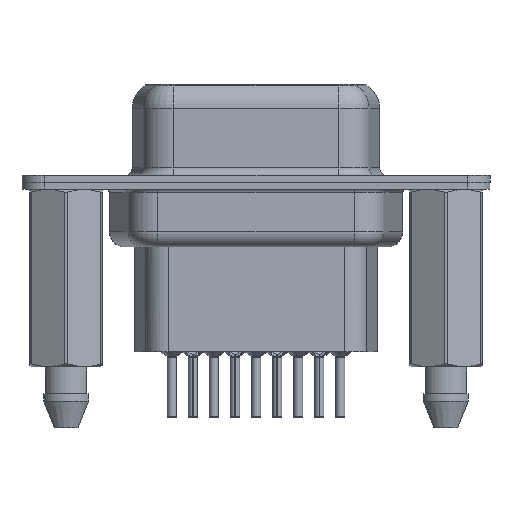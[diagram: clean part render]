
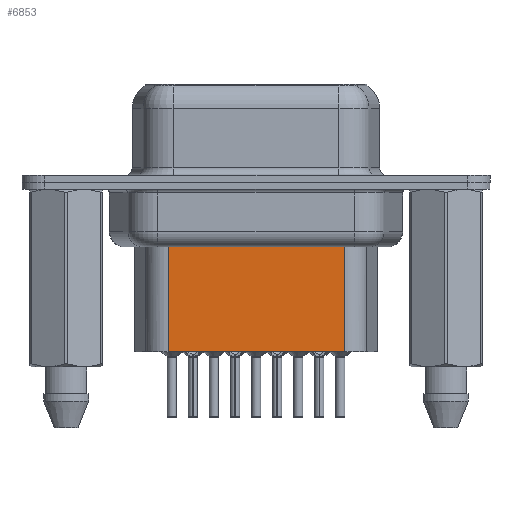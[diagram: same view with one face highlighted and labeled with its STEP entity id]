
A CAD part, front view. The second image highlights one B-rep face of the part: STEP entity #6853.
In plain terms, the highlighted planar face has unit normal (0, -1, 0).
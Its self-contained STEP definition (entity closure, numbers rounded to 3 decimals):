
#758 = CARTESIAN_POINT ( 'NONE',  ( 6.706, -3.5, -4.097 ) ) ;
#928 = CARTESIAN_POINT ( 'NONE',  ( 6.706, -3.5, -3.1 ) ) ;
#2281 = EDGE_CURVE ( 'NONE', #19360, #7440, #21546, .T. ) ;
#2859 = AXIS2_PLACEMENT_3D ( 'NONE', #928, #18677, #21998 ) ;
#3710 = ORIENTED_EDGE ( 'NONE', *, *, #4539, .T. ) ;
#3723 = DIRECTION ( 'NONE',  ( -1., 0., 0. ) ) ;
#4539 = EDGE_CURVE ( 'NONE', #7440, #18703, #18444, .T. ) ;
#6853 = ADVANCED_FACE ( 'NONE', ( #16727 ), #15343, .T. ) ;
#7440 = VERTEX_POINT ( 'NONE', #758 ) ;
#7667 = LINE ( 'NONE', #19545, #13420 ) ;
#11241 = CARTESIAN_POINT ( 'NONE',  ( 6.706, -3.5, -11.15 ) ) ;
#12076 = VECTOR ( 'NONE', #21766, 1000. ) ;
#12569 = VERTEX_POINT ( 'NONE', #12985 ) ;
#12985 = CARTESIAN_POINT ( 'NONE',  ( 18.294, -3.5, -11.15 ) ) ;
#13420 = VECTOR ( 'NONE', #3723, 1000. ) ;
#14421 = DIRECTION ( 'NONE',  ( -1., 0., 0. ) ) ;
#14539 = CARTESIAN_POINT ( 'NONE',  ( 6.459, -3.5, -4.097 ) ) ;
#15077 = VECTOR ( 'NONE', #14421, 1000. ) ;
#15098 = ORIENTED_EDGE ( 'NONE', *, *, #2281, .T. ) ;
#15343 = PLANE ( 'NONE',  #2859 ) ;
#16295 = VECTOR ( 'NONE', #19643, 1000. ) ;
#16582 = EDGE_CURVE ( 'NONE', #19360, #12569, #19754, .T. ) ;
#16727 = FACE_OUTER_BOUND ( 'NONE', #22612, .T. ) ;
#17377 = ORIENTED_EDGE ( 'NONE', *, *, #16582, .F. ) ;
#18444 = LINE ( 'NONE', #18986, #12076 ) ;
#18601 = EDGE_CURVE ( 'NONE', #12569, #18703, #7667, .T. ) ;
#18677 = DIRECTION ( 'NONE',  ( 0., -1., 0. ) ) ;
#18703 = VERTEX_POINT ( 'NONE', #11241 ) ;
#18986 = CARTESIAN_POINT ( 'NONE',  ( 6.706, -3.5, -3.1 ) ) ;
#19360 = VERTEX_POINT ( 'NONE', #22179 ) ;
#19545 = CARTESIAN_POINT ( 'NONE',  ( 6.706, -3.5, -11.15 ) ) ;
#19643 = DIRECTION ( 'NONE',  ( 0., 0., -1. ) ) ;
#19754 = LINE ( 'NONE', #21457, #16295 ) ;
#19840 = ORIENTED_EDGE ( 'NONE', *, *, #18601, .F. ) ;
#21457 = CARTESIAN_POINT ( 'NONE',  ( 18.294, -3.5, -3.1 ) ) ;
#21546 = LINE ( 'NONE', #14539, #15077 ) ;
#21766 = DIRECTION ( 'NONE',  ( 0., 0., -1. ) ) ;
#21998 = DIRECTION ( 'NONE',  ( 1., 0., 0. ) ) ;
#22179 = CARTESIAN_POINT ( 'NONE',  ( 18.294, -3.5, -4.097 ) ) ;
#22612 = EDGE_LOOP ( 'NONE', ( #17377, #15098, #3710, #19840 ) ) ;
